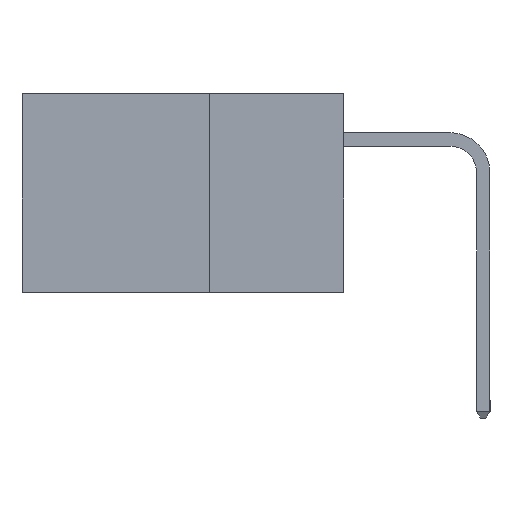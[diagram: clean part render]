
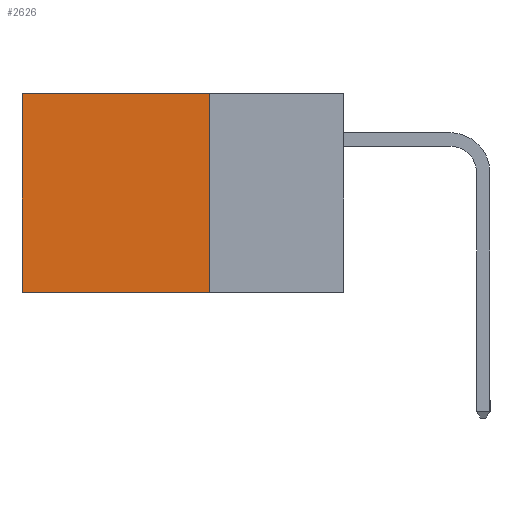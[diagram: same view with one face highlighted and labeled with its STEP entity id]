
A CAD part, left-side view. The second image highlights one B-rep face of the part: STEP entity #2626.
In plain terms, the highlighted planar face has unit normal (-1, 0, 0).
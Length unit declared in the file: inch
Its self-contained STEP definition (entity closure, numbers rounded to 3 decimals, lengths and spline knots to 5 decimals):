
#32 = EDGE_CURVE ( 'NONE', #9776, #8707, #7145, .T. ) ;
#719 = DIRECTION ( 'NONE',  ( 0., 0., -1. ) ) ;
#1087 = CARTESIAN_POINT ( 'NONE',  ( 0.2615, 0.25, -0.37 ) ) ;
#2194 = ORIENTED_EDGE ( 'NONE', *, *, #12677, .F. ) ;
#2198 = EDGE_CURVE ( 'NONE', #8707, #14626, #9601, .T. ) ;
#2301 = CARTESIAN_POINT ( 'NONE',  ( 0.2615, 0.6, -0.37 ) ) ;
#2626 = ADVANCED_FACE ( 'NONE', ( #12385 ), #7211, .F. ) ;
#2650 = VECTOR ( 'NONE', #9839, 39.37008 ) ;
#2656 = DIRECTION ( 'NONE',  ( 0., 0., -1. ) ) ;
#3048 = LINE ( 'NONE', #1087, #2650 ) ;
#3389 = VECTOR ( 'NONE', #10137, 39.37008 ) ;
#4051 = VERTEX_POINT ( 'NONE', #12636 ) ;
#5823 = VECTOR ( 'NONE', #719, 39.37008 ) ;
#6230 = AXIS2_PLACEMENT_3D ( 'NONE', #6913, #6626, #6588 ) ;
#6588 = DIRECTION ( 'NONE',  ( 0., 0., -1. ) ) ;
#6626 = DIRECTION ( 'NONE',  ( 1., 0., 0. ) ) ;
#6913 = CARTESIAN_POINT ( 'NONE',  ( 0.2615, 0.25, -0.37 ) ) ;
#7145 = LINE ( 'NONE', #10597, #3389 ) ;
#7181 = ORIENTED_EDGE ( 'NONE', *, *, #2198, .T. ) ;
#7211 = PLANE ( 'NONE',  #6230 ) ;
#8707 = VERTEX_POINT ( 'NONE', #9494 ) ;
#9485 = ORIENTED_EDGE ( 'NONE', *, *, #32, .T. ) ;
#9494 = CARTESIAN_POINT ( 'NONE',  ( 0.2615, 0.6, 0. ) ) ;
#9601 = LINE ( 'NONE', #2301, #12763 ) ;
#9776 = VERTEX_POINT ( 'NONE', #13363 ) ;
#9839 = DIRECTION ( 'NONE',  ( 0., 1., 0. ) ) ;
#10137 = DIRECTION ( 'NONE',  ( 0., 1., 0. ) ) ;
#10570 = EDGE_LOOP ( 'NONE', ( #7181, #14650, #2194, #9485 ) ) ;
#10597 = CARTESIAN_POINT ( 'NONE',  ( 0.2615, 0.25, 0. ) ) ;
#10894 = CARTESIAN_POINT ( 'NONE',  ( 0.2615, 0.6, -0.37 ) ) ;
#11616 = EDGE_CURVE ( 'NONE', #4051, #14626, #3048, .T. ) ;
#11851 = LINE ( 'NONE', #15359, #5823 ) ;
#12385 = FACE_OUTER_BOUND ( 'NONE', #10570, .T. ) ;
#12636 = CARTESIAN_POINT ( 'NONE',  ( 0.2615, 0.25, -0.37 ) ) ;
#12677 = EDGE_CURVE ( 'NONE', #9776, #4051, #11851, .T. ) ;
#12763 = VECTOR ( 'NONE', #2656, 39.37008 ) ;
#13363 = CARTESIAN_POINT ( 'NONE',  ( 0.2615, 0.25, 0. ) ) ;
#14626 = VERTEX_POINT ( 'NONE', #10894 ) ;
#14650 = ORIENTED_EDGE ( 'NONE', *, *, #11616, .F. ) ;
#15359 = CARTESIAN_POINT ( 'NONE',  ( 0.2615, 0.25, -0.37 ) ) ;
